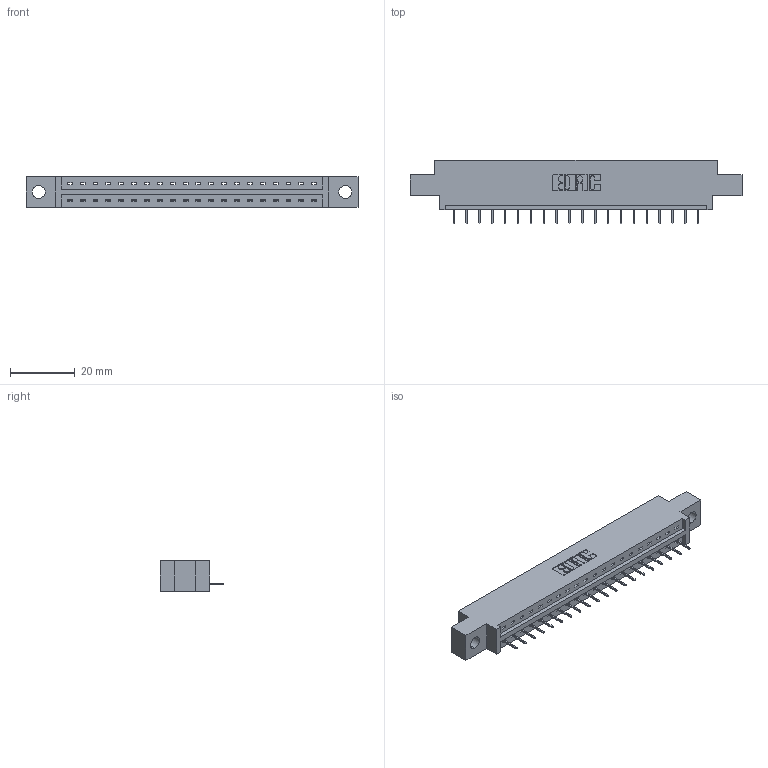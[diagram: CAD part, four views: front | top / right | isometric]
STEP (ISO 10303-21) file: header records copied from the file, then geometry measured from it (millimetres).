
FILE_DESCRIPTION (( 'STEP AP203' ), '1' );
FILE_NAME ('337-020-524-604.STEP', '2018-08-05T08:56:11', ( '' ), ( '' ), 'SwSTEP 2.0', 'SolidWorks 2016', '' );
FILE_SCHEMA (( 'CONFIG_CONTROL_DESIGN' ));
Length unit declared in the file: inch
Products named in the file (3): 337 Part_0.170 Offset - 0.156 Dia-TH; 345-292-001_345-293-124; 337-020-524-604
Assembly tree (21 placements, depth 2):
  337-020-524-604
    337 Part_0.170 Offset - 0.156 Dia-TH
    345-292-001_345-293-124  x20
Bounding box: 102.26 x 19.69 x 9.4 mm (x, y, z)
Volume: 10068.6 mm3; surface area: 9896.2 mm2
Topology: 21 solids, 21 shells, 1438 faces, 4163 edges, 2694 vertices
Faces by surface type: plane 1114, cylinder 324
Entity records: 17921 total; most frequent: CARTESIAN_POINT 3126, ORIENTED_EDGE 3082, DIRECTION 2677, EDGE_CURVE 1541, VECTOR 1417, LINE 1417, VERTEX_POINT 1022, AXIS2_PLACEMENT_3D 630
